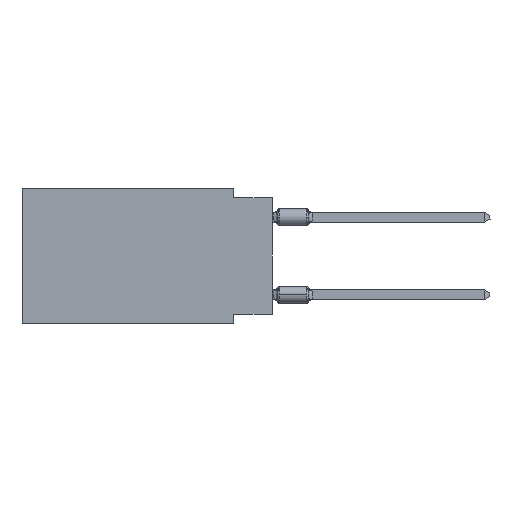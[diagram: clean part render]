
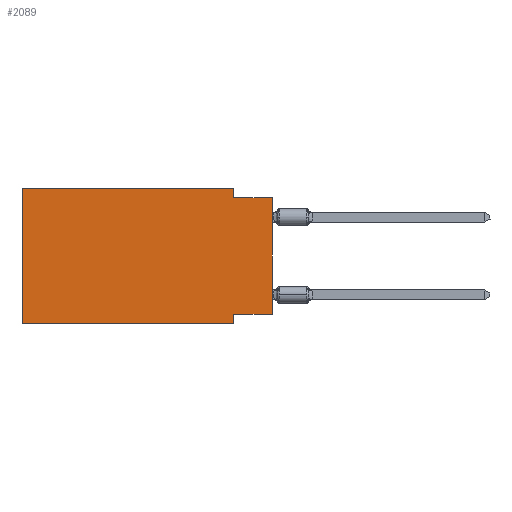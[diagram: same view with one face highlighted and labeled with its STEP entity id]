
A CAD part, left-side view. The second image highlights one B-rep face of the part: STEP entity #2089.
In plain terms, the highlighted planar face has unit normal (-1, 0, 0).
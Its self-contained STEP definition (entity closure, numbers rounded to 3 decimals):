
#1207 = EDGE_CURVE ( 'NONE', #31276, #7145, #25391, .T. ) ;
#1619 = CARTESIAN_POINT ( 'NONE',  ( 0., 16.383, 0. ) ) ;
#1716 = EDGE_CURVE ( 'NONE', #6182, #5961, #20347, .T. ) ;
#2089 = ADVANCED_FACE ( 'NONE', ( #34241 ), #34044, .F. ) ;
#2241 = CARTESIAN_POINT ( 'NONE',  ( 0., 0., -0.635 ) ) ;
#2880 = VERTEX_POINT ( 'NONE', #15809 ) ;
#3095 = DIRECTION ( 'NONE',  ( 0., 0., -1. ) ) ;
#3776 = CARTESIAN_POINT ( 'NONE',  ( 0., 0., -8.255 ) ) ;
#4238 = CARTESIAN_POINT ( 'NONE',  ( 0., 16.383, -8.89 ) ) ;
#4412 = VECTOR ( 'NONE', #20882, 1000. ) ;
#4423 = VECTOR ( 'NONE', #6082, 1000. ) ;
#5684 = CARTESIAN_POINT ( 'NONE',  ( 0., 16.383, 0. ) ) ;
#5961 = VERTEX_POINT ( 'NONE', #21878 ) ;
#6082 = DIRECTION ( 'NONE',  ( 0., -1., 0. ) ) ;
#6182 = VERTEX_POINT ( 'NONE', #4238 ) ;
#7145 = VERTEX_POINT ( 'NONE', #2241 ) ;
#7546 = LINE ( 'NONE', #1619, #4412 ) ;
#7621 = EDGE_CURVE ( 'NONE', #31276, #28676, #33541, .T. ) ;
#7803 = DIRECTION ( 'NONE',  ( 0., 0., 1. ) ) ;
#8218 = LINE ( 'NONE', #33985, #27380 ) ;
#8638 = DIRECTION ( 'NONE',  ( 1., 0., 0. ) ) ;
#10363 = CARTESIAN_POINT ( 'NONE',  ( 0., 0., -8.255 ) ) ;
#11369 = VECTOR ( 'NONE', #27353, 1000. ) ;
#11570 = VERTEX_POINT ( 'NONE', #22295 ) ;
#11872 = ORIENTED_EDGE ( 'NONE', *, *, #1716, .T. ) ;
#12400 = VECTOR ( 'NONE', #16485, 1000. ) ;
#12919 = LINE ( 'NONE', #21793, #11369 ) ;
#14305 = ORIENTED_EDGE ( 'NONE', *, *, #1207, .T. ) ;
#14595 = CARTESIAN_POINT ( 'NONE',  ( 0., 2.54, 0. ) ) ;
#14610 = CARTESIAN_POINT ( 'NONE',  ( 0., 16.383, -8.89 ) ) ;
#14723 = EDGE_CURVE ( 'NONE', #11570, #36012, #7546, .T. ) ;
#15809 = CARTESIAN_POINT ( 'NONE',  ( 0., 2.54, -0.635 ) ) ;
#16485 = DIRECTION ( 'NONE',  ( 0., 1., 0. ) ) ;
#16727 = DIRECTION ( 'NONE',  ( 0., -1., 0. ) ) ;
#18853 = EDGE_LOOP ( 'NONE', ( #14305, #32994, #21128, #25384, #24132, #11872, #32377, #26825 ) ) ;
#19120 = CARTESIAN_POINT ( 'NONE',  ( 0., 2.54, -8.255 ) ) ;
#19929 = DIRECTION ( 'NONE',  ( 0., 0., -1. ) ) ;
#20347 = LINE ( 'NONE', #14610, #4423 ) ;
#20882 = DIRECTION ( 'NONE',  ( 0., -1., 0. ) ) ;
#21128 = ORIENTED_EDGE ( 'NONE', *, *, #33574, .F. ) ;
#21793 = CARTESIAN_POINT ( 'NONE',  ( 0., 2.54, -8.89 ) ) ;
#21878 = CARTESIAN_POINT ( 'NONE',  ( 0., 2.54, -8.89 ) ) ;
#22295 = CARTESIAN_POINT ( 'NONE',  ( 0., 16.383, 0. ) ) ;
#22923 = DIRECTION ( 'NONE',  ( 0., 0., 1. ) ) ;
#23317 = VECTOR ( 'NONE', #22923, 1000. ) ;
#24132 = ORIENTED_EDGE ( 'NONE', *, *, #30810, .F. ) ;
#25343 = LINE ( 'NONE', #14595, #25571 ) ;
#25384 = ORIENTED_EDGE ( 'NONE', *, *, #14723, .F. ) ;
#25391 = LINE ( 'NONE', #27991, #34626 ) ;
#25571 = VECTOR ( 'NONE', #3095, 1000. ) ;
#26825 = ORIENTED_EDGE ( 'NONE', *, *, #7621, .F. ) ;
#27353 = DIRECTION ( 'NONE',  ( 0., 0., -1. ) ) ;
#27380 = VECTOR ( 'NONE', #16727, 1000. ) ;
#27920 = LINE ( 'NONE', #5684, #23317 ) ;
#27991 = CARTESIAN_POINT ( 'NONE',  ( 0., 0., 0. ) ) ;
#28676 = VERTEX_POINT ( 'NONE', #19120 ) ;
#30810 = EDGE_CURVE ( 'NONE', #6182, #11570, #27920, .T. ) ;
#31062 = CARTESIAN_POINT ( 'NONE',  ( 0., 16.383, 0. ) ) ;
#31276 = VERTEX_POINT ( 'NONE', #3776 ) ;
#32377 = ORIENTED_EDGE ( 'NONE', *, *, #33830, .F. ) ;
#32994 = ORIENTED_EDGE ( 'NONE', *, *, #34512, .F. ) ;
#33541 = LINE ( 'NONE', #10363, #12400 ) ;
#33574 = EDGE_CURVE ( 'NONE', #36012, #2880, #25343, .T. ) ;
#33830 = EDGE_CURVE ( 'NONE', #28676, #5961, #12919, .T. ) ;
#33985 = CARTESIAN_POINT ( 'NONE',  ( 0., 0., -0.635 ) ) ;
#34044 = PLANE ( 'NONE',  #34672 ) ;
#34241 = FACE_OUTER_BOUND ( 'NONE', #18853, .T. ) ;
#34512 = EDGE_CURVE ( 'NONE', #2880, #7145, #8218, .T. ) ;
#34626 = VECTOR ( 'NONE', #7803, 1000. ) ;
#34672 = AXIS2_PLACEMENT_3D ( 'NONE', #31062, #8638, #19929 ) ;
#36012 = VERTEX_POINT ( 'NONE', #36412 ) ;
#36412 = CARTESIAN_POINT ( 'NONE',  ( 0., 2.54, 0. ) ) ;
